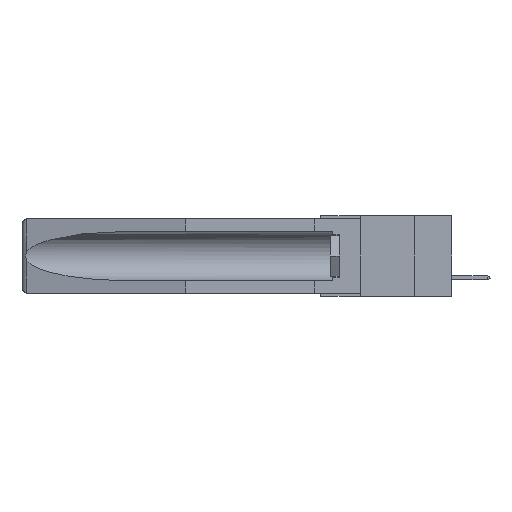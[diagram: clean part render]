
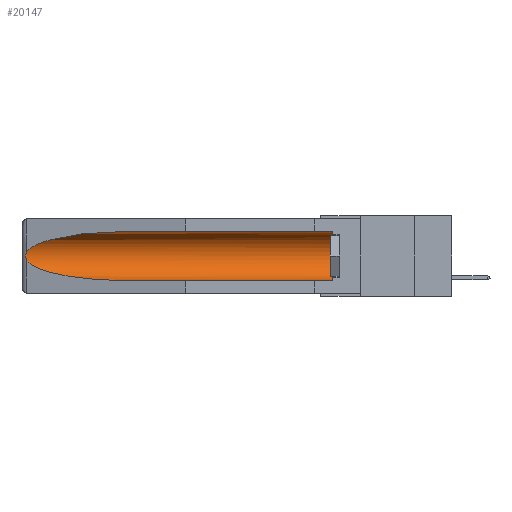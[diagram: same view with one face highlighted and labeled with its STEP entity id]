
A CAD part, left-side view. The second image highlights one B-rep face of the part: STEP entity #20147.
In plain terms, the highlighted cylindrical face has radius 2.857 mm (diameter 5.715 mm), a partial arc.
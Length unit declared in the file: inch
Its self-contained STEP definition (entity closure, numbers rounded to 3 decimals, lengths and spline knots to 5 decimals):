
#390 = VECTOR ( 'NONE', #21071, 39.37008 ) ;
#2061 = CARTESIAN_POINT ( 'NONE',  ( 0.2675, 1.53308, -0.17534 ) ) ;
#2574 = CARTESIAN_POINT ( 'NONE',  ( 0.21114, 1.30732, -0.284 ) ) ;
#2605 = VERTEX_POINT ( 'NONE', #5423 ) ;
#3062 = CARTESIAN_POINT ( 'NONE',  ( 0.26537, 1.52718, -0.14972 ) ) ;
#3122 = EDGE_CURVE ( 'NONE', #11897, #7594, #16887, .T. ) ;
#4459 = CARTESIAN_POINT ( 'NONE',  ( 0.2673, 1.53269, -0.17917 ) ) ;
#4543 =( BOUNDED_CURVE ( )  B_SPLINE_CURVE ( 3, ( #10250, #19856, #24672, #3062 ),
 .UNSPECIFIED., .F., .F. ) 
 B_SPLINE_CURVE_WITH_KNOTS ( ( 4, 4 ),
 ( 4.71239, 6.08839 ),
 .UNSPECIFIED. ) 
 CURVE ( )  GEOMETRIC_REPRESENTATION_ITEM ( )  RATIONAL_B_SPLINE_CURVE ( ( 1., 0.848, 0.848, 1. ) ) 
 REPRESENTATION_ITEM ( '' )  );
#5423 = CARTESIAN_POINT ( 'NONE',  ( 0.155, 0.126, -0.284 ) ) ;
#5565 = ORIENTED_EDGE ( 'NONE', *, *, #29529, .F. ) ;
#5834 = VERTEX_POINT ( 'NONE', #9775 ) ;
#6613 = EDGE_CURVE ( 'NONE', #5834, #7177, #4543, .T. ) ;
#7177 = VERTEX_POINT ( 'NONE', #9063 ) ;
#7232 = ORIENTED_EDGE ( 'NONE', *, *, #6613, .T. ) ;
#7455 = CARTESIAN_POINT ( 'NONE',  ( 0.155, 0.126, -0.1715 ) ) ;
#7594 = VERTEX_POINT ( 'NONE', #10568 ) ;
#7829 = ORIENTED_EDGE ( 'NONE', *, *, #10112, .T. ) ;
#7859 = CARTESIAN_POINT ( 'NONE',  ( 0.26537, 1.52718, -0.19328 ) ) ;
#8236 = EDGE_CURVE ( 'NONE', #2605, #21171, #28583, .T. ) ;
#8858 = AXIS2_PLACEMENT_3D ( 'NONE', #7455, #24075, #26665 ) ;
#9063 = CARTESIAN_POINT ( 'NONE',  ( 0.26537, 1.52718, -0.14972 ) ) ;
#9143 = CARTESIAN_POINT ( 'NONE',  ( 0.2673, 1.5327, -0.16383 ) ) ;
#9187 = CARTESIAN_POINT ( 'NONE',  ( 0.155, -0.30754, -0.1715 ) ) ;
#9305 = DIRECTION ( 'NONE',  ( 0., 1., 0. ) ) ;
#9751 = ORIENTED_EDGE ( 'NONE', *, *, #3122, .T. ) ;
#9775 = CARTESIAN_POINT ( 'NONE',  ( 0.155, 1.07973, -0.059 ) ) ;
#10112 = EDGE_CURVE ( 'NONE', #7177, #11897, #14299, .T. ) ;
#10250 = CARTESIAN_POINT ( 'NONE',  ( 0.155, 1.07973, -0.059 ) ) ;
#10568 = CARTESIAN_POINT ( 'NONE',  ( 0.155, 1.07973, -0.284 ) ) ;
#11461 = CARTESIAN_POINT ( 'NONE',  ( 0.155, -0.30754, -0.059 ) ) ;
#11630 = DIRECTION ( 'NONE',  ( 0., 1., 0. ) ) ;
#11897 = VERTEX_POINT ( 'NONE', #7859 ) ;
#11902 = CARTESIAN_POINT ( 'NONE',  ( 0.26654, 1.53092, -0.15636 ) ) ;
#13662 = CYLINDRICAL_SURFACE ( 'NONE', #19971, 0.1125 ) ;
#14207 = VECTOR ( 'NONE', #9305, 39.37008 ) ;
#14236 = EDGE_CURVE ( 'NONE', #21171, #5834, #17514, .T. ) ;
#14299 = B_SPLINE_CURVE_WITH_KNOTS ( 'NONE', 3,
 ( #26152, #30608, #11902, #9143, #30512, #2061, #4459, #21062, #23473, #19338 ),
 .UNSPECIFIED., .F., .F.,
 ( 4, 2, 2, 2, 4 ),
 ( 0., 0.00029, 0.00058, 0.00087, 0.00117 ),
 .UNSPECIFIED. ) ;
#14390 = CARTESIAN_POINT ( 'NONE',  ( 0.25451, 1.48313, -0.24835 ) ) ;
#16887 =( BOUNDED_CURVE ( )  B_SPLINE_CURVE ( 3, ( #28650, #14390, #2574, #23997 ),
 .UNSPECIFIED., .F., .F. ) 
 B_SPLINE_CURVE_WITH_KNOTS ( ( 4, 4 ),
 ( 0.1948, 1.5708 ),
 .UNSPECIFIED. ) 
 CURVE ( )  GEOMETRIC_REPRESENTATION_ITEM ( )  RATIONAL_B_SPLINE_CURVE ( ( 1., 0.848, 0.848, 1. ) ) 
 REPRESENTATION_ITEM ( '' )  );
#17406 = ORIENTED_EDGE ( 'NONE', *, *, #14236, .T. ) ;
#17514 = LINE ( 'NONE', #11461, #14207 ) ;
#18294 = CARTESIAN_POINT ( 'NONE',  ( 0.155, 0.126, -0.059 ) ) ;
#19338 = CARTESIAN_POINT ( 'NONE',  ( 0.26537, 1.52718, -0.19328 ) ) ;
#19856 = CARTESIAN_POINT ( 'NONE',  ( 0.21114, 1.30732, -0.059 ) ) ;
#19971 = AXIS2_PLACEMENT_3D ( 'NONE', #9187, #11630, #25790 ) ;
#20147 = ADVANCED_FACE ( 'NONE', ( #27810 ), #13662, .F. ) ;
#20879 = EDGE_LOOP ( 'NONE', ( #7232, #7829, #9751, #5565, #22694, #17406 ) ) ;
#21062 = CARTESIAN_POINT ( 'NONE',  ( 0.26655, 1.53094, -0.18657 ) ) ;
#21071 = DIRECTION ( 'NONE',  ( 0., 1., 0. ) ) ;
#21171 = VERTEX_POINT ( 'NONE', #18294 ) ;
#22694 = ORIENTED_EDGE ( 'NONE', *, *, #8236, .T. ) ;
#23473 = CARTESIAN_POINT ( 'NONE',  ( 0.26597, 1.5296, -0.19026 ) ) ;
#23583 = CARTESIAN_POINT ( 'NONE',  ( 0.155, -0.30754, -0.284 ) ) ;
#23997 = CARTESIAN_POINT ( 'NONE',  ( 0.155, 1.07973, -0.284 ) ) ;
#24075 = DIRECTION ( 'NONE',  ( 0., -1., 0. ) ) ;
#24672 = CARTESIAN_POINT ( 'NONE',  ( 0.25451, 1.48313, -0.09465 ) ) ;
#25790 = DIRECTION ( 'NONE',  ( 0., 0., 1. ) ) ;
#26152 = CARTESIAN_POINT ( 'NONE',  ( 0.26537, 1.52718, -0.14972 ) ) ;
#26665 = DIRECTION ( 'NONE',  ( 0., 0., 1. ) ) ;
#27810 = FACE_OUTER_BOUND ( 'NONE', #20879, .T. ) ;
#28583 = CIRCLE ( 'NONE', #8858, 0.1125 ) ;
#28650 = CARTESIAN_POINT ( 'NONE',  ( 0.26537, 1.52718, -0.19328 ) ) ;
#29039 = LINE ( 'NONE', #23583, #390 ) ;
#29529 = EDGE_CURVE ( 'NONE', #2605, #7594, #29039, .T. ) ;
#30512 = CARTESIAN_POINT ( 'NONE',  ( 0.2675, 1.53308, -0.16763 ) ) ;
#30608 = CARTESIAN_POINT ( 'NONE',  ( 0.26597, 1.52961, -0.15275 ) ) ;
